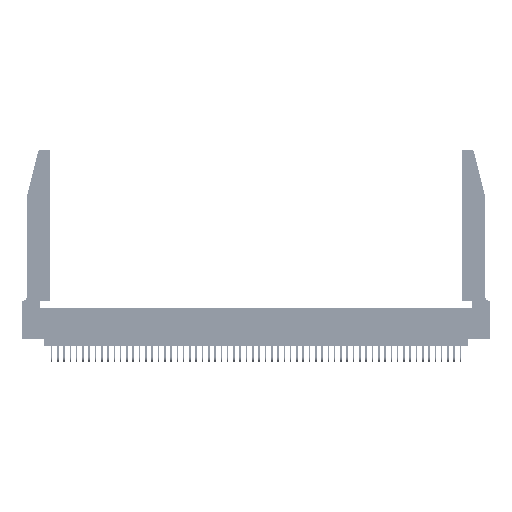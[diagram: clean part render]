
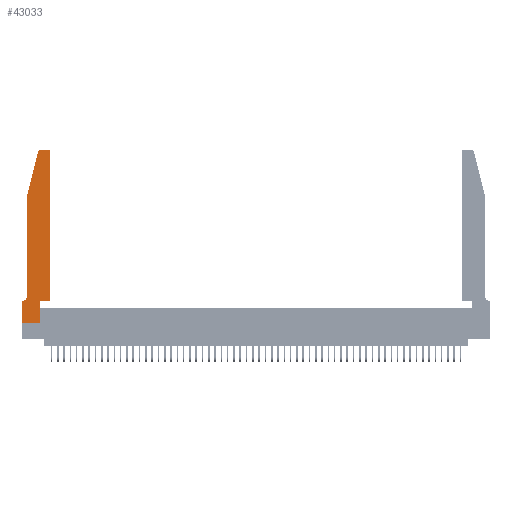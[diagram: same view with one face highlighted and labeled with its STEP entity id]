
A CAD part, top view. The second image highlights one B-rep face of the part: STEP entity #43033.
In plain terms, the highlighted planar face has unit normal (0, 0, 1).
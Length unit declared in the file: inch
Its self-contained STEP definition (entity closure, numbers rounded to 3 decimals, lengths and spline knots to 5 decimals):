
#484 = DIRECTION ( 'NONE',  ( 1., 0., 0. ) ) ;
#909 = CARTESIAN_POINT ( 'NONE',  ( 0., 0., 0.37 ) ) ;
#1025 = AXIS2_PLACEMENT_3D ( 'NONE', #12249, #29358, #46523 ) ;
#1151 = CARTESIAN_POINT ( 'NONE',  ( 0.0755, 2., 0.37 ) ) ;
#1334 = DIRECTION ( 'NONE',  ( -1., 0., 0. ) ) ;
#1948 = CARTESIAN_POINT ( 'NONE',  ( 0.0755, 2., 0.37 ) ) ;
#2325 = VERTEX_POINT ( 'NONE', #17787 ) ;
#2403 = CARTESIAN_POINT ( 'NONE',  ( 0.4205, 2.75, 0.37 ) ) ;
#2457 = LINE ( 'NONE', #55128, #49116 ) ;
#2678 = LINE ( 'NONE', #33255, #33320 ) ;
#3445 = DIRECTION ( 'NONE',  ( 1., 0., 0. ) ) ;
#3606 = VERTEX_POINT ( 'NONE', #17268 ) ;
#3871 = DIRECTION ( 'NONE',  ( -1., 0., 0. ) ) ;
#4606 = CARTESIAN_POINT ( 'NONE',  ( 0.2865, 0.35, 0.37 ) ) ;
#4822 = VECTOR ( 'NONE', #51531, 39.37008 ) ;
#5219 = CARTESIAN_POINT ( 'NONE',  ( 0.0055, 0.35, 0.37 ) ) ;
#6791 = CARTESIAN_POINT ( 'NONE',  ( 0., 0., 0.37 ) ) ;
#7002 = EDGE_LOOP ( 'NONE', ( #34100, #9352, #22835, #33048, #48801, #8253, #11427, #12927, #29502, #36590, #13311, #45379 ) ) ;
#7152 = VERTEX_POINT ( 'NONE', #4606 ) ;
#8253 = ORIENTED_EDGE ( 'NONE', *, *, #13455, .T. ) ;
#8542 = VERTEX_POINT ( 'NONE', #2403 ) ;
#8988 = EDGE_CURVE ( 'NONE', #18117, #2325, #51598, .T. ) ;
#9084 = VERTEX_POINT ( 'NONE', #24062 ) ;
#9352 = ORIENTED_EDGE ( 'NONE', *, *, #43815, .T. ) ;
#9895 = EDGE_CURVE ( 'NONE', #25643, #7152, #33457, .T. ) ;
#11427 = ORIENTED_EDGE ( 'NONE', *, *, #43165, .T. ) ;
#12249 = CARTESIAN_POINT ( 'NONE',  ( 0., 0.35, 0.37 ) ) ;
#12781 = FACE_OUTER_BOUND ( 'NONE', #7002, .T. ) ;
#12927 = ORIENTED_EDGE ( 'NONE', *, *, #14539, .T. ) ;
#13311 = ORIENTED_EDGE ( 'NONE', *, *, #42022, .T. ) ;
#13455 = EDGE_CURVE ( 'NONE', #36843, #9084, #2457, .T. ) ;
#14151 = DIRECTION ( 'NONE',  ( 0., 0., -1. ) ) ;
#14539 = EDGE_CURVE ( 'NONE', #48125, #25643, #43846, .T. ) ;
#14790 = CARTESIAN_POINT ( 'NONE',  ( 0.284, 2.72, 0.37 ) ) ;
#15332 = DIRECTION ( 'NONE',  ( 1., 0., 0. ) ) ;
#16638 = AXIS2_PLACEMENT_3D ( 'NONE', #30874, #14151, #1334 ) ;
#17206 = CARTESIAN_POINT ( 'NONE',  ( 0., 0., 0.37 ) ) ;
#17268 = CARTESIAN_POINT ( 'NONE',  ( 0.284, 2.75, 0.37 ) ) ;
#17787 = CARTESIAN_POINT ( 'NONE',  ( 0.0755, 0.42, 0.37 ) ) ;
#18117 = VERTEX_POINT ( 'NONE', #1948 ) ;
#18150 = CARTESIAN_POINT ( 'NONE',  ( 0.25487, 2.72718, 0.37 ) ) ;
#18213 = VECTOR ( 'NONE', #39523, 39.37008 ) ;
#21749 = CARTESIAN_POINT ( 'NONE',  ( 0.4505, 0.35, 0.37 ) ) ;
#21928 = DIRECTION ( 'NONE',  ( 1., 0., 0. ) ) ;
#21976 = EDGE_CURVE ( 'NONE', #35596, #8542, #52950, .T. ) ;
#22835 = ORIENTED_EDGE ( 'NONE', *, *, #44949, .T. ) ;
#24062 = CARTESIAN_POINT ( 'NONE',  ( 0., 0.35, 0.37 ) ) ;
#25077 = PLANE ( 'NONE',  #1025 ) ;
#25494 = DIRECTION ( 'NONE',  ( -1., 0., 0. ) ) ;
#25643 = VERTEX_POINT ( 'NONE', #46136 ) ;
#26442 = DIRECTION ( 'NONE',  ( -0.239, -0.971, 0. ) ) ;
#27457 = CARTESIAN_POINT ( 'NONE',  ( 0.0755, 2., 0.37 ) ) ;
#28359 = DIRECTION ( 'NONE',  ( 0., 0., 1. ) ) ;
#29358 = DIRECTION ( 'NONE',  ( 0., 0., 1. ) ) ;
#29502 = ORIENTED_EDGE ( 'NONE', *, *, #9895, .T. ) ;
#30874 = CARTESIAN_POINT ( 'NONE',  ( 0.0055, 0.42, 0.37 ) ) ;
#32877 = LINE ( 'NONE', #35029, #18213 ) ;
#33048 = ORIENTED_EDGE ( 'NONE', *, *, #8988, .T. ) ;
#33255 = CARTESIAN_POINT ( 'NONE',  ( 0.2605, 2.75, 0.37 ) ) ;
#33320 = VECTOR ( 'NONE', #3871, 39.37008 ) ;
#33457 = LINE ( 'NONE', #54962, #38810 ) ;
#33756 = CARTESIAN_POINT ( 'NONE',  ( 0.4205, 2.72, 0.37 ) ) ;
#34100 = ORIENTED_EDGE ( 'NONE', *, *, #34573, .T. ) ;
#34573 = EDGE_CURVE ( 'NONE', #8542, #3606, #2678, .T. ) ;
#35029 = CARTESIAN_POINT ( 'NONE',  ( 0.4505, 0.35, 0.37 ) ) ;
#35596 = VERTEX_POINT ( 'NONE', #54778 ) ;
#36590 = ORIENTED_EDGE ( 'NONE', *, *, #52426, .T. ) ;
#36843 = VERTEX_POINT ( 'NONE', #5219 ) ;
#37256 = DIRECTION ( 'NONE',  ( 0., 1., 0. ) ) ;
#37497 = DIRECTION ( 'NONE',  ( 0., 0., 1. ) ) ;
#38100 = AXIS2_PLACEMENT_3D ( 'NONE', #14790, #28359, #15332 ) ;
#38637 = VECTOR ( 'NONE', #26442, 39.37008 ) ;
#38810 = VECTOR ( 'NONE', #37256, 39.37008 ) ;
#39523 = DIRECTION ( 'NONE',  ( 0., 1., 0. ) ) ;
#39614 = VERTEX_POINT ( 'NONE', #43161 ) ;
#39683 = LINE ( 'NONE', #21749, #42365 ) ;
#40225 = VERTEX_POINT ( 'NONE', #18150 ) ;
#42022 = EDGE_CURVE ( 'NONE', #39614, #35596, #32877, .T. ) ;
#42365 = VECTOR ( 'NONE', #21928, 39.37008 ) ;
#42612 = EDGE_CURVE ( 'NONE', #2325, #36843, #54838, .T. ) ;
#43033 = ADVANCED_FACE ( 'NONE', ( #12781 ), #25077, .T. ) ;
#43161 = CARTESIAN_POINT ( 'NONE',  ( 0.4505, 0.35, 0.37 ) ) ;
#43165 = EDGE_CURVE ( 'NONE', #9084, #48125, #49447, .T. ) ;
#43815 = EDGE_CURVE ( 'NONE', #3606, #40225, #44029, .T. ) ;
#43846 = LINE ( 'NONE', #17206, #50502 ) ;
#44029 = CIRCLE ( 'NONE', #38100, 0.03 ) ;
#44949 = EDGE_CURVE ( 'NONE', #40225, #18117, #51328, .T. ) ;
#45379 = ORIENTED_EDGE ( 'NONE', *, *, #21976, .T. ) ;
#46136 = CARTESIAN_POINT ( 'NONE',  ( 0.2865, 0., 0.37 ) ) ;
#46523 = DIRECTION ( 'NONE',  ( 1., 0., 0. ) ) ;
#48125 = VERTEX_POINT ( 'NONE', #6791 ) ;
#48801 = ORIENTED_EDGE ( 'NONE', *, *, #42612, .T. ) ;
#49116 = VECTOR ( 'NONE', #25494, 39.37008 ) ;
#49150 = AXIS2_PLACEMENT_3D ( 'NONE', #33756, #37497, #3445 ) ;
#49447 = LINE ( 'NONE', #909, #4822 ) ;
#50502 = VECTOR ( 'NONE', #484, 39.37008 ) ;
#51328 = LINE ( 'NONE', #1151, #38637 ) ;
#51531 = DIRECTION ( 'NONE',  ( 0., -1., 0. ) ) ;
#51598 = LINE ( 'NONE', #27457, #54910 ) ;
#52426 = EDGE_CURVE ( 'NONE', #7152, #39614, #39683, .T. ) ;
#52950 = CIRCLE ( 'NONE', #49150, 0.03 ) ;
#53003 = DIRECTION ( 'NONE',  ( 0., -1., 0. ) ) ;
#54778 = CARTESIAN_POINT ( 'NONE',  ( 0.4505, 2.72, 0.37 ) ) ;
#54838 = CIRCLE ( 'NONE', #16638, 0.07 ) ;
#54910 = VECTOR ( 'NONE', #53003, 39.37008 ) ;
#54962 = CARTESIAN_POINT ( 'NONE',  ( 0.2865, 0.35, 0.37 ) ) ;
#55128 = CARTESIAN_POINT ( 'NONE',  ( 0.0755, 0.35, 0.37 ) ) ;
